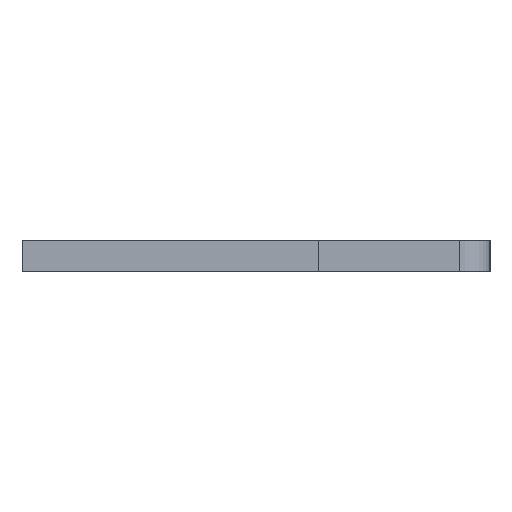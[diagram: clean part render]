
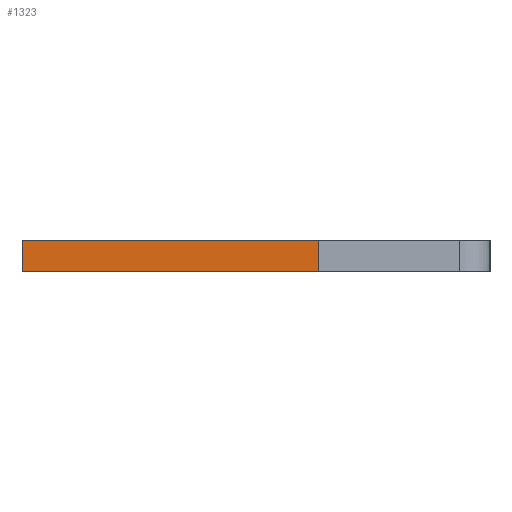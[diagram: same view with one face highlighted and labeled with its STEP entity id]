
A CAD part, left-side view. The second image highlights one B-rep face of the part: STEP entity #1323.
In plain terms, the highlighted face is planar.
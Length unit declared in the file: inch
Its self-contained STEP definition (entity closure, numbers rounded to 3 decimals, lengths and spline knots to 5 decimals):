
#86 = LINE ( 'NONE', #349, #808 ) ;
#107 = CARTESIAN_POINT ( 'NONE',  ( -0.01, 0.15, -0.04 ) ) ;
#169 = VERTEX_POINT ( 'NONE', #829 ) ;
#172 = VERTEX_POINT ( 'NONE', #1051 ) ;
#220 = CARTESIAN_POINT ( 'NONE',  ( 0.01, 0.15, -0.04 ) ) ;
#226 = DIRECTION ( 'NONE',  ( -1., 0., 0. ) ) ;
#233 = DIRECTION ( 'NONE',  ( 0., 1., 0. ) ) ;
#249 = DIRECTION ( 'NONE',  ( 0., 0., 1. ) ) ;
#282 = EDGE_LOOP ( 'NONE', ( #427, #739, #574, #1008 ) ) ;
#349 = CARTESIAN_POINT ( 'NONE',  ( 0.01, 0.15, -0.04 ) ) ;
#355 = CARTESIAN_POINT ( 'NONE',  ( -0.01, 0.15, -0.04 ) ) ;
#360 = PLANE ( 'NONE',  #807 ) ;
#365 = CARTESIAN_POINT ( 'NONE',  ( 0.01, -0.04, -0.04 ) ) ;
#401 = EDGE_CURVE ( 'NONE', #1436, #172, #1388, .T. ) ;
#422 = LINE ( 'NONE', #220, #869 ) ;
#427 = ORIENTED_EDGE ( 'NONE', *, *, #939, .T. ) ;
#565 = DIRECTION ( 'NONE',  ( 0., 1., 0. ) ) ;
#574 = ORIENTED_EDGE ( 'NONE', *, *, #1020, .F. ) ;
#601 = CARTESIAN_POINT ( 'NONE',  ( 0.01, -0.04, -0.04 ) ) ;
#712 = DIRECTION ( 'NONE',  ( 1., 0., 0. ) ) ;
#739 = ORIENTED_EDGE ( 'NONE', *, *, #958, .F. ) ;
#807 = AXIS2_PLACEMENT_3D ( 'NONE', #1072, #249, #712 ) ;
#808 = VECTOR ( 'NONE', #565, 39.37008 ) ;
#829 = CARTESIAN_POINT ( 'NONE',  ( 0.01, 0.15, -0.04 ) ) ;
#869 = VECTOR ( 'NONE', #226, 39.37008 ) ;
#939 = EDGE_CURVE ( 'NONE', #172, #1070, #1419, .T. ) ;
#946 = DIRECTION ( 'NONE',  ( -1., 0., 0. ) ) ;
#958 = EDGE_CURVE ( 'NONE', #169, #1070, #422, .T. ) ;
#967 = VECTOR ( 'NONE', #946, 39.37008 ) ;
#1008 = ORIENTED_EDGE ( 'NONE', *, *, #401, .T. ) ;
#1020 = EDGE_CURVE ( 'NONE', #1436, #169, #86, .T. ) ;
#1051 = CARTESIAN_POINT ( 'NONE',  ( -0.01, -0.04, -0.04 ) ) ;
#1070 = VERTEX_POINT ( 'NONE', #355 ) ;
#1072 = CARTESIAN_POINT ( 'NONE',  ( 0.01, 0.15, -0.04 ) ) ;
#1079 = FACE_OUTER_BOUND ( 'NONE', #282, .T. ) ;
#1202 = VECTOR ( 'NONE', #233, 39.37008 ) ;
#1323 = ADVANCED_FACE ( 'NONE', ( #1079 ), #360, .F. ) ;
#1388 = LINE ( 'NONE', #601, #967 ) ;
#1419 = LINE ( 'NONE', #107, #1202 ) ;
#1436 = VERTEX_POINT ( 'NONE', #365 ) ;
